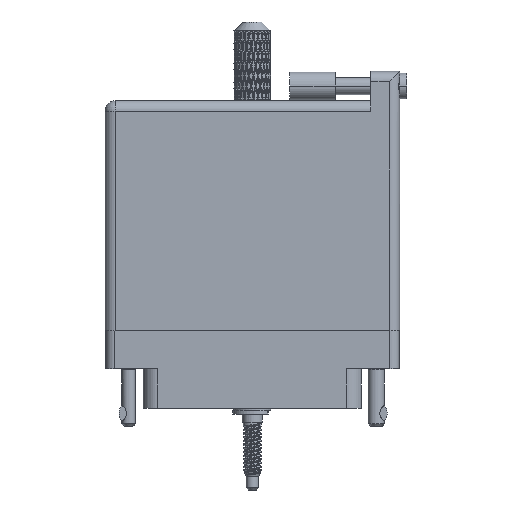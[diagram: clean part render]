
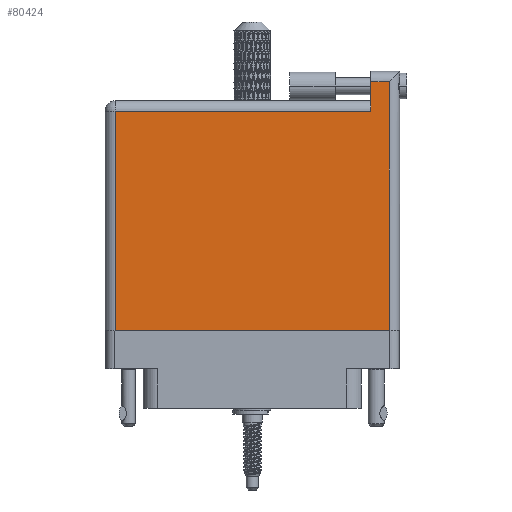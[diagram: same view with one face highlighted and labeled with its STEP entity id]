
A CAD part, front view. The second image highlights one B-rep face of the part: STEP entity #80424.
In plain terms, the highlighted face is planar.
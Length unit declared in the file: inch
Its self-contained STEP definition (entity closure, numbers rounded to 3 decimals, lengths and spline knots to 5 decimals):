
#2049 = VECTOR ( 'NONE', #87811, 39.37008 ) ;
#2915 = CARTESIAN_POINT ( 'NONE',  ( 0.07, 0., 0. ) ) ;
#3441 = LINE ( 'NONE', #19905, #2049 ) ;
#3848 = DIRECTION ( 'NONE',  ( 0., 1., 0. ) ) ;
#4051 = DIRECTION ( 'NONE',  ( -1., 0., 0. ) ) ;
#7642 = CARTESIAN_POINT ( 'NONE',  ( 0.07, 1.496, 0. ) ) ;
#8614 = PLANE ( 'NONE',  #106792 ) ;
#8989 = DIRECTION ( 'NONE',  ( 0., 0., -1. ) ) ;
#12338 = EDGE_CURVE ( 'NONE', #97437, #70946, #50263, .T. ) ;
#12865 = CARTESIAN_POINT ( 'NONE',  ( 0., 1.496, 0. ) ) ;
#19184 = CARTESIAN_POINT ( 'NONE',  ( 0.07, 0., 0. ) ) ;
#19905 = CARTESIAN_POINT ( 'NONE',  ( 0., 1.696, 0. ) ) ;
#20416 = CARTESIAN_POINT ( 'NONE',  ( 1.938, 1.696, 0. ) ) ;
#21175 = EDGE_LOOP ( 'NONE', ( #36469, #56878, #41016, #42832, #100929, #107807 ) ) ;
#26204 = LINE ( 'NONE', #105379, #104494 ) ;
#32545 = VERTEX_POINT ( 'NONE', #65873 ) ;
#35790 = EDGE_CURVE ( 'NONE', #87240, #32545, #63905, .T. ) ;
#36469 = ORIENTED_EDGE ( 'NONE', *, *, #12338, .T. ) ;
#39438 = FACE_OUTER_BOUND ( 'NONE', #21175, .T. ) ;
#40698 = VECTOR ( 'NONE', #4051, 39.37008 ) ;
#41016 = ORIENTED_EDGE ( 'NONE', *, *, #74499, .T. ) ;
#42832 = ORIENTED_EDGE ( 'NONE', *, *, #35790, .T. ) ;
#46477 = CARTESIAN_POINT ( 'NONE',  ( 1.811, 1.766, 0. ) ) ;
#50263 = LINE ( 'NONE', #63180, #67625 ) ;
#53394 = DIRECTION ( 'NONE',  ( 0., -1., 0. ) ) ;
#53842 = DIRECTION ( 'NONE',  ( 1., 0., 0. ) ) ;
#56878 = ORIENTED_EDGE ( 'NONE', *, *, #92147, .T. ) ;
#60676 = CARTESIAN_POINT ( 'NONE',  ( 0., 1.566, 0. ) ) ;
#62883 = DIRECTION ( 'NONE',  ( 0., -1., 0. ) ) ;
#63180 = CARTESIAN_POINT ( 'NONE',  ( 0., 0., 0. ) ) ;
#63764 = CARTESIAN_POINT ( 'NONE',  ( 1.938, 0., 0. ) ) ;
#63905 = LINE ( 'NONE', #46477, #83714 ) ;
#65873 = CARTESIAN_POINT ( 'NONE',  ( 1.811, 1.496, 0. ) ) ;
#66033 = LINE ( 'NONE', #12865, #40698 ) ;
#67284 = VECTOR ( 'NONE', #53394, 39.37008 ) ;
#67625 = VECTOR ( 'NONE', #53842, 39.37008 ) ;
#70946 = VERTEX_POINT ( 'NONE', #63764 ) ;
#73482 = VERTEX_POINT ( 'NONE', #7642 ) ;
#74499 = EDGE_CURVE ( 'NONE', #96083, #87240, #3441, .T. ) ;
#80424 = ADVANCED_FACE ( 'NONE', ( #39438 ), #8614, .F. ) ;
#83714 = VECTOR ( 'NONE', #62883, 39.37008 ) ;
#87240 = VERTEX_POINT ( 'NONE', #103583 ) ;
#87811 = DIRECTION ( 'NONE',  ( -1., 0., 0. ) ) ;
#92147 = EDGE_CURVE ( 'NONE', #70946, #96083, #26204, .T. ) ;
#95044 = LINE ( 'NONE', #19184, #67284 ) ;
#96083 = VERTEX_POINT ( 'NONE', #20416 ) ;
#97343 = EDGE_CURVE ( 'NONE', #73482, #97437, #95044, .T. ) ;
#97437 = VERTEX_POINT ( 'NONE', #2915 ) ;
#97442 = EDGE_CURVE ( 'NONE', #32545, #73482, #66033, .T. ) ;
#100929 = ORIENTED_EDGE ( 'NONE', *, *, #97442, .T. ) ;
#102419 = DIRECTION ( 'NONE',  ( -1., 0., 0. ) ) ;
#103583 = CARTESIAN_POINT ( 'NONE',  ( 1.811, 1.696, 0. ) ) ;
#104494 = VECTOR ( 'NONE', #3848, 39.37008 ) ;
#105379 = CARTESIAN_POINT ( 'NONE',  ( 1.938, 1.766, 0. ) ) ;
#106792 = AXIS2_PLACEMENT_3D ( 'NONE', #60676, #8989, #102419 ) ;
#107807 = ORIENTED_EDGE ( 'NONE', *, *, #97343, .T. ) ;
